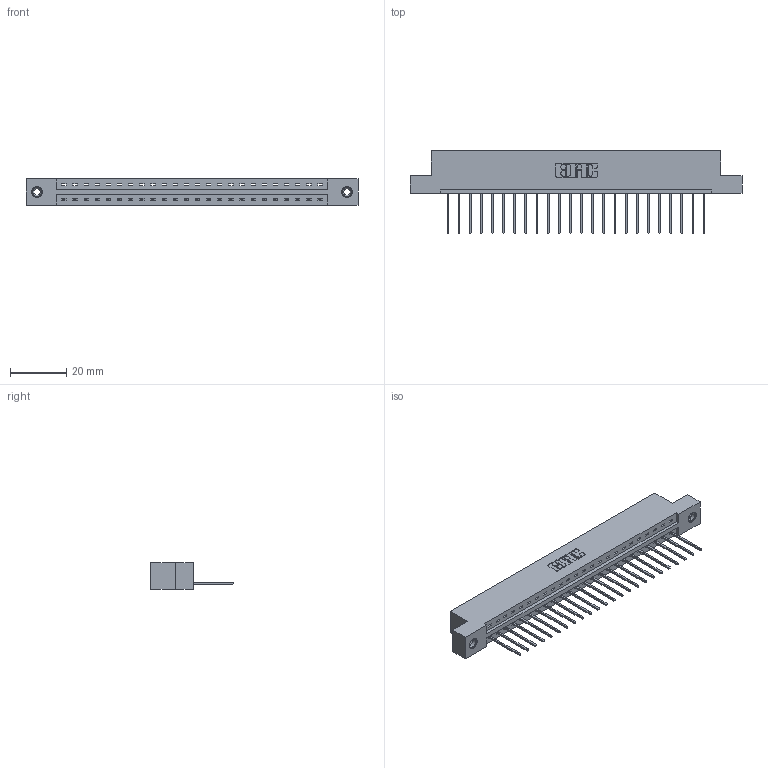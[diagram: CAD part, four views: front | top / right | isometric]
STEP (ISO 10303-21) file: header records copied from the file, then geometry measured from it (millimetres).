
FILE_DESCRIPTION (( 'STEP AP203' ), '1' );
FILE_NAME ('337-024-540-108.STEP', '2018-08-05T19:45:34', ( '' ), ( '' ), 'SwSTEP 2.0', 'SolidWorks 2016', '' );
FILE_SCHEMA (( 'CONFIG_CONTROL_DESIGN' ));
Length unit declared in the file: inch
Products named in the file (4): 345-250-001_345-250-003-102; 337-024-540-108; 337 Part_Flush Mounting Lugs - 0.156 Dia-TI; 345-292-001_345-293-140
Assembly tree (27 placements, depth 2):
  337-024-540-108
    337 Part_Flush Mounting Lugs - 0.156 Dia-TI
    345-292-001_345-293-140  x24
    345-250-001_345-250-003-102  x2
Bounding box: 118.11 x 29.47 x 9.4 mm (x, y, z)
Volume: 12076.3 mm3; surface area: 12650.1 mm2
Topology: 27 solids, 27 shells, 1662 faces, 4959 edges, 3266 vertices
Faces by surface type: plane 1206, cylinder 440, cone 12, torus 4
Entity records: 21372 total; most frequent: CARTESIAN_POINT 3701, ORIENTED_EDGE 3654, DIRECTION 3185, EDGE_CURVE 1827, VECTOR 1679, LINE 1679, VERTEX_POINT 1212, AXIS2_PLACEMENT_3D 753
